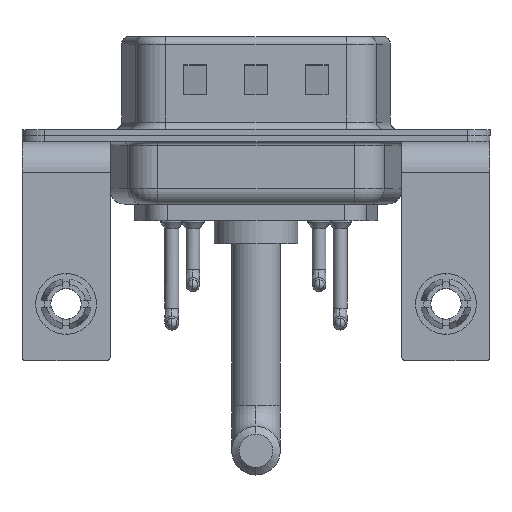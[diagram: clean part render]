
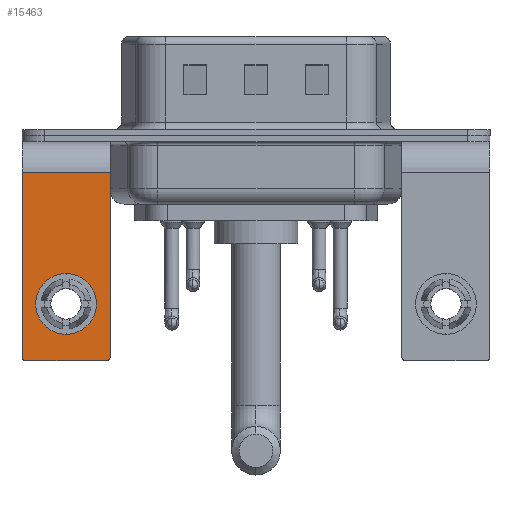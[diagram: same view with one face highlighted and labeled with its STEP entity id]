
A CAD part, front view. The second image highlights one B-rep face of the part: STEP entity #15463.
In plain terms, the highlighted planar face has unit normal (0, -1, 0).
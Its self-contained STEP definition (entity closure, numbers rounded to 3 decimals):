
#237 = CARTESIAN_POINT ( 'NONE',  ( 0., -6.25, -13.07 ) ) ;
#1488 = VERTEX_POINT ( 'NONE', #14328 ) ;
#1993 = ORIENTED_EDGE ( 'NONE', *, *, #9305, .T. ) ;
#3137 = EDGE_CURVE ( 'NONE', #13715, #18136, #19290, .T. ) ;
#3822 = CARTESIAN_POINT ( 'NONE',  ( 0., -6.25, -9.07 ) ) ;
#3872 = VERTEX_POINT ( 'NONE', #17816 ) ;
#3881 = DIRECTION ( 'NONE',  ( -1., 0., 0. ) ) ;
#3991 = AXIS2_PLACEMENT_3D ( 'NONE', #14114, #12350, #17254 ) ;
#4373 = DIRECTION ( 'NONE',  ( 0., 0., 1. ) ) ;
#4663 = LINE ( 'NONE', #7890, #15057 ) ;
#5042 = LINE ( 'NONE', #20665, #17843 ) ;
#5652 = DIRECTION ( 'NONE',  ( 0., 0., 1. ) ) ;
#5793 = CIRCLE ( 'NONE', #20314, 2. ) ;
#5870 = EDGE_LOOP ( 'NONE', ( #8605, #1993, #20942, #8360, #11890, #8735 ) ) ;
#6116 = CARTESIAN_POINT ( 'NONE',  ( -2.65, -6.25, -14.55 ) ) ;
#6979 = DIRECTION ( 'NONE',  ( 0., 1., 0. ) ) ;
#7049 = FACE_OUTER_BOUND ( 'NONE', #5870, .T. ) ;
#7167 = VERTEX_POINT ( 'NONE', #3822 ) ;
#7558 = AXIS2_PLACEMENT_3D ( 'NONE', #13404, #6979, #15408 ) ;
#7602 = CARTESIAN_POINT ( 'NONE',  ( 2.65, -6.25, -14.55 ) ) ;
#7890 = CARTESIAN_POINT ( 'NONE',  ( -2.9, -6.25, -2.4 ) ) ;
#8360 = ORIENTED_EDGE ( 'NONE', *, *, #20004, .T. ) ;
#8448 = DIRECTION ( 'NONE',  ( 0., -1., 0. ) ) ;
#8473 = CARTESIAN_POINT ( 'NONE',  ( 2.9, -6.25, -2.4 ) ) ;
#8605 = ORIENTED_EDGE ( 'NONE', *, *, #19347, .T. ) ;
#8735 = ORIENTED_EDGE ( 'NONE', *, *, #9218, .T. ) ;
#9218 = EDGE_CURVE ( 'NONE', #13250, #3872, #19419, .T. ) ;
#9276 = AXIS2_PLACEMENT_3D ( 'NONE', #6116, #8448, #18320 ) ;
#9305 = EDGE_CURVE ( 'NONE', #1488, #18136, #13529, .T. ) ;
#9480 = DIRECTION ( 'NONE',  ( 0., -1., 0. ) ) ;
#10037 = DIRECTION ( 'NONE',  ( 0., 0., -1. ) ) ;
#10249 = ORIENTED_EDGE ( 'NONE', *, *, #10827, .T. ) ;
#10491 = FACE_BOUND ( 'NONE', #18623, .T. ) ;
#10827 = EDGE_CURVE ( 'NONE', #19457, #7167, #5793, .T. ) ;
#10836 = VERTEX_POINT ( 'NONE', #17536 ) ;
#10895 = CARTESIAN_POINT ( 'NONE',  ( 2.9, -6.25, -2.4 ) ) ;
#11225 = DIRECTION ( 'NONE',  ( -1., 0., 0. ) ) ;
#11336 = EDGE_CURVE ( 'NONE', #13250, #10836, #5042, .T. ) ;
#11890 = ORIENTED_EDGE ( 'NONE', *, *, #11336, .F. ) ;
#12350 = DIRECTION ( 'NONE',  ( 0., 1., 0. ) ) ;
#13217 = CIRCLE ( 'NONE', #7558, 2. ) ;
#13250 = VERTEX_POINT ( 'NONE', #8473 ) ;
#13404 = CARTESIAN_POINT ( 'NONE',  ( 0., -6.25, -11.07 ) ) ;
#13529 = CIRCLE ( 'NONE', #9276, 0.25 ) ;
#13715 = VERTEX_POINT ( 'NONE', #15609 ) ;
#13787 = PLANE ( 'NONE',  #3991 ) ;
#14114 = CARTESIAN_POINT ( 'NONE',  ( 2.9, -6.25, -2.4 ) ) ;
#14328 = CARTESIAN_POINT ( 'NONE',  ( -2.9, -6.25, -14.55 ) ) ;
#14641 = DIRECTION ( 'NONE',  ( 0., 0., -1. ) ) ;
#15057 = VECTOR ( 'NONE', #14641, 1000. ) ;
#15391 = ORIENTED_EDGE ( 'NONE', *, *, #16228, .T. ) ;
#15408 = DIRECTION ( 'NONE',  ( 0., 0., 1. ) ) ;
#15441 = AXIS2_PLACEMENT_3D ( 'NONE', #7602, #9480, #4373 ) ;
#15463 = ADVANCED_FACE ( 'NONE', ( #10491, #7049 ), #13787, .F. ) ;
#15537 = CARTESIAN_POINT ( 'NONE',  ( 2.9, -6.25, -14.8 ) ) ;
#15609 = CARTESIAN_POINT ( 'NONE',  ( 2.65, -6.25, -14.8 ) ) ;
#15652 = VECTOR ( 'NONE', #11225, 1000. ) ;
#16228 = EDGE_CURVE ( 'NONE', #7167, #19457, #13217, .T. ) ;
#17254 = DIRECTION ( 'NONE',  ( 0., 0., 1. ) ) ;
#17536 = CARTESIAN_POINT ( 'NONE',  ( 2.9, -6.25, -14.55 ) ) ;
#17551 = CIRCLE ( 'NONE', #15441, 0.25 ) ;
#17816 = CARTESIAN_POINT ( 'NONE',  ( -2.9, -6.25, -2.4 ) ) ;
#17843 = VECTOR ( 'NONE', #10037, 1000. ) ;
#18136 = VERTEX_POINT ( 'NONE', #21899 ) ;
#18159 = VECTOR ( 'NONE', #3881, 1000. ) ;
#18320 = DIRECTION ( 'NONE',  ( 0., 0., 1. ) ) ;
#18623 = EDGE_LOOP ( 'NONE', ( #10249, #15391 ) ) ;
#19290 = LINE ( 'NONE', #15537, #18159 ) ;
#19347 = EDGE_CURVE ( 'NONE', #3872, #1488, #4663, .T. ) ;
#19419 = LINE ( 'NONE', #10895, #15652 ) ;
#19457 = VERTEX_POINT ( 'NONE', #237 ) ;
#20004 = EDGE_CURVE ( 'NONE', #13715, #10836, #17551, .T. ) ;
#20314 = AXIS2_PLACEMENT_3D ( 'NONE', #20838, #20621, #5652 ) ;
#20621 = DIRECTION ( 'NONE',  ( 0., 1., 0. ) ) ;
#20665 = CARTESIAN_POINT ( 'NONE',  ( 2.9, -6.25, -2.4 ) ) ;
#20838 = CARTESIAN_POINT ( 'NONE',  ( 0., -6.25, -11.07 ) ) ;
#20942 = ORIENTED_EDGE ( 'NONE', *, *, #3137, .F. ) ;
#21899 = CARTESIAN_POINT ( 'NONE',  ( -2.65, -6.25, -14.8 ) ) ;
